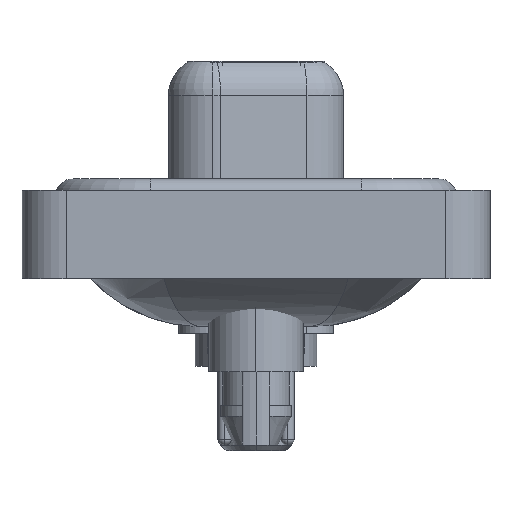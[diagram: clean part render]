
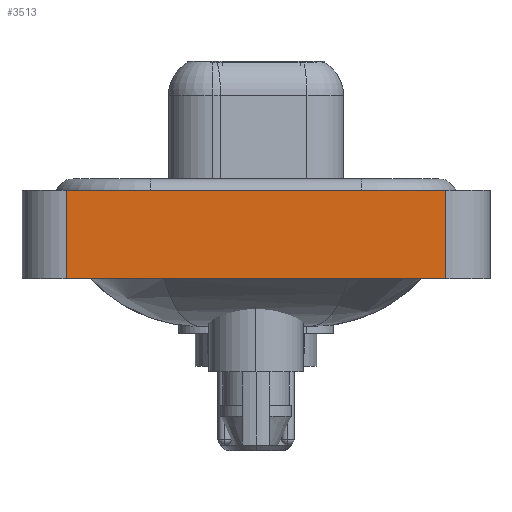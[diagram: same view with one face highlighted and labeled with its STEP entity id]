
A CAD part, left-side view. The second image highlights one B-rep face of the part: STEP entity #3513.
In plain terms, the highlighted planar face has unit normal (-1, 0, 0).
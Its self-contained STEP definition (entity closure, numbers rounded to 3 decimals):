
#382 = CARTESIAN_POINT ( 'NONE',  ( -7.3, -8.55, 0.4 ) ) ;
#624 = CARTESIAN_POINT ( 'NONE',  ( -7.3, 8.55, -3.6 ) ) ;
#1278 = VECTOR ( 'NONE', #20566, 1000. ) ;
#3513 = ADVANCED_FACE ( 'NONE', ( #4556 ), #17052, .T. ) ;
#3670 = VERTEX_POINT ( 'NONE', #22293 ) ;
#4556 = FACE_OUTER_BOUND ( 'NONE', #17054, .T. ) ;
#5477 = ORIENTED_EDGE ( 'NONE', *, *, #9140, .F. ) ;
#5952 = DIRECTION ( 'NONE',  ( 0., -1., 0. ) ) ;
#6813 = VERTEX_POINT ( 'NONE', #7446 ) ;
#7446 = CARTESIAN_POINT ( 'NONE',  ( -7.3, -8.55, 0.4 ) ) ;
#7466 = DIRECTION ( 'NONE',  ( 0., 0., 1. ) ) ;
#7707 = DIRECTION ( 'NONE',  ( 0., -1., 0. ) ) ;
#7862 = LINE ( 'NONE', #11828, #14117 ) ;
#8756 = CARTESIAN_POINT ( 'NONE',  ( -7.3, -8.55, -3.6 ) ) ;
#9140 = EDGE_CURVE ( 'NONE', #12055, #3670, #13733, .T. ) ;
#10844 = AXIS2_PLACEMENT_3D ( 'NONE', #11872, #22911, #7466 ) ;
#10853 = CARTESIAN_POINT ( 'NONE',  ( -7.3, -8.55, -3.6 ) ) ;
#10986 = EDGE_CURVE ( 'NONE', #12055, #15993, #7862, .T. ) ;
#11048 = ORIENTED_EDGE ( 'NONE', *, *, #19339, .T. ) ;
#11485 = EDGE_CURVE ( 'NONE', #3670, #6813, #16838, .T. ) ;
#11828 = CARTESIAN_POINT ( 'NONE',  ( -7.3, -8.55, -3.6 ) ) ;
#11872 = CARTESIAN_POINT ( 'NONE',  ( -7.3, -8.55, -3.6 ) ) ;
#12055 = VERTEX_POINT ( 'NONE', #12464 ) ;
#12464 = CARTESIAN_POINT ( 'NONE',  ( -7.3, 8.55, -3.6 ) ) ;
#13733 = LINE ( 'NONE', #624, #1278 ) ;
#14117 = VECTOR ( 'NONE', #5952, 1000. ) ;
#14536 = VECTOR ( 'NONE', #7707, 1000. ) ;
#15886 = VECTOR ( 'NONE', #18197, 1000. ) ;
#15993 = VERTEX_POINT ( 'NONE', #8756 ) ;
#16153 = ORIENTED_EDGE ( 'NONE', *, *, #10986, .T. ) ;
#16838 = LINE ( 'NONE', #382, #14536 ) ;
#17052 = PLANE ( 'NONE',  #10844 ) ;
#17054 = EDGE_LOOP ( 'NONE', ( #11048, #19038, #5477, #16153 ) ) ;
#18197 = DIRECTION ( 'NONE',  ( 0., 0., 1. ) ) ;
#19038 = ORIENTED_EDGE ( 'NONE', *, *, #11485, .F. ) ;
#19339 = EDGE_CURVE ( 'NONE', #15993, #6813, #19992, .T. ) ;
#19992 = LINE ( 'NONE', #10853, #15886 ) ;
#20566 = DIRECTION ( 'NONE',  ( 0., 0., 1. ) ) ;
#22293 = CARTESIAN_POINT ( 'NONE',  ( -7.3, 8.55, 0.4 ) ) ;
#22911 = DIRECTION ( 'NONE',  ( -1., 0., 0. ) ) ;
